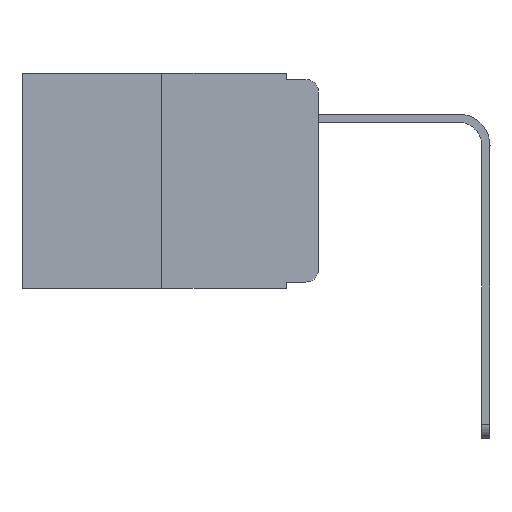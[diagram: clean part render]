
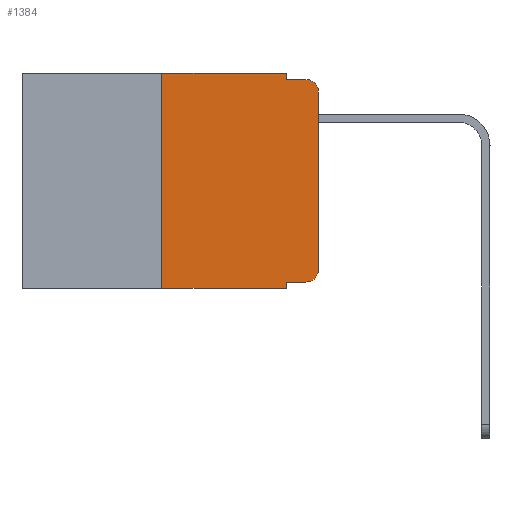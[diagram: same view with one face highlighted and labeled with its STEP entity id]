
A CAD part, left-side view. The second image highlights one B-rep face of the part: STEP entity #1384.
In plain terms, the highlighted planar face has unit normal (-1, 0, 0).
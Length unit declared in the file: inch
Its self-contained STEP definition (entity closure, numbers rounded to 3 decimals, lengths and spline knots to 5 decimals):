
#184 = ORIENTED_EDGE ( 'NONE', *, *, #1946, .T. ) ;
#216 = VERTEX_POINT ( 'NONE', #1196 ) ;
#349 = DIRECTION ( 'NONE',  ( 0., 0., -1. ) ) ;
#419 = CARTESIAN_POINT ( 'NONE',  ( 0., 0.25, 0. ) ) ;
#544 = ORIENTED_EDGE ( 'NONE', *, *, #1931, .F. ) ;
#556 = EDGE_CURVE ( 'NONE', #3804, #8467, #6731, .T. ) ;
#856 = LINE ( 'NONE', #9484, #6596 ) ;
#1089 = CARTESIAN_POINT ( 'NONE',  ( 0., 0., -0.313 ) ) ;
#1102 = DIRECTION ( 'NONE',  ( -1., 0., 0. ) ) ;
#1115 = DIRECTION ( 'NONE',  ( 0., 0., 1. ) ) ;
#1196 = CARTESIAN_POINT ( 'NONE',  ( 0., 0.051, -0.333 ) ) ;
#1223 = CARTESIAN_POINT ( 'NONE',  ( 0., 0.051, -0.01 ) ) ;
#1312 = CARTESIAN_POINT ( 'NONE',  ( 0., 0.25, -0.343 ) ) ;
#1384 = ADVANCED_FACE ( 'NONE', ( #4943 ), #7823, .F. ) ;
#1387 = LINE ( 'NONE', #9319, #8066 ) ;
#1457 = EDGE_CURVE ( 'NONE', #3573, #3804, #7039, .T. ) ;
#1873 = DIRECTION ( 'NONE',  ( 0., 0., -1. ) ) ;
#1931 = EDGE_CURVE ( 'NONE', #4893, #8467, #4245, .T. ) ;
#1946 = EDGE_CURVE ( 'NONE', #6320, #6126, #856, .T. ) ;
#2114 = VECTOR ( 'NONE', #9587, 39.37008 ) ;
#2255 = LINE ( 'NONE', #8440, #7183 ) ;
#2430 = VECTOR ( 'NONE', #4287, 39.37008 ) ;
#3028 = VECTOR ( 'NONE', #3867, 39.37008 ) ;
#3076 = EDGE_CURVE ( 'NONE', #216, #4515, #8195, .T. ) ;
#3193 = VERTEX_POINT ( 'NONE', #8867 ) ;
#3284 = CARTESIAN_POINT ( 'NONE',  ( 0., 0.02, -0.313 ) ) ;
#3522 = EDGE_CURVE ( 'NONE', #3193, #4893, #1387, .T. ) ;
#3533 = ORIENTED_EDGE ( 'NONE', *, *, #5985, .F. ) ;
#3573 = VERTEX_POINT ( 'NONE', #1089 ) ;
#3605 = CARTESIAN_POINT ( 'NONE',  ( 0., 0., -0.03 ) ) ;
#3804 = VERTEX_POINT ( 'NONE', #3605 ) ;
#3867 = DIRECTION ( 'NONE',  ( 0., -1., 0. ) ) ;
#3978 = ORIENTED_EDGE ( 'NONE', *, *, #4857, .F. ) ;
#4219 = DIRECTION ( 'NONE',  ( 0., 0., 1. ) ) ;
#4245 = LINE ( 'NONE', #9513, #2114 ) ;
#4287 = DIRECTION ( 'NONE',  ( 0., -1., 0. ) ) ;
#4418 = CARTESIAN_POINT ( 'NONE',  ( 0., 0.02, -0.333 ) ) ;
#4446 = ORIENTED_EDGE ( 'NONE', *, *, #7745, .T. ) ;
#4467 = ORIENTED_EDGE ( 'NONE', *, *, #3522, .F. ) ;
#4511 = CARTESIAN_POINT ( 'NONE',  ( 0., 0.02, -0.03 ) ) ;
#4515 = VERTEX_POINT ( 'NONE', #4418 ) ;
#4616 = ORIENTED_EDGE ( 'NONE', *, *, #9634, .F. ) ;
#4785 = LINE ( 'NONE', #6127, #3028 ) ;
#4789 = CARTESIAN_POINT ( 'NONE',  ( 0., 0.25, 0. ) ) ;
#4812 = DIRECTION ( 'NONE',  ( 1., 0., 0. ) ) ;
#4857 = EDGE_CURVE ( 'NONE', #6320, #6624, #4986, .T. ) ;
#4861 = CARTESIAN_POINT ( 'NONE',  ( 0., 0.051, -0.343 ) ) ;
#4893 = VERTEX_POINT ( 'NONE', #1223 ) ;
#4932 = CARTESIAN_POINT ( 'NONE',  ( 0., 0., 0. ) ) ;
#4943 = FACE_OUTER_BOUND ( 'NONE', #7488, .T. ) ;
#4986 = LINE ( 'NONE', #419, #6398 ) ;
#5155 = CIRCLE ( 'NONE', #8229, 0.02 ) ;
#5441 = ORIENTED_EDGE ( 'NONE', *, *, #556, .T. ) ;
#5495 = DIRECTION ( 'NONE',  ( 0., 0., -1. ) ) ;
#5796 = DIRECTION ( 'NONE',  ( 0., -1., 0. ) ) ;
#5985 = EDGE_CURVE ( 'NONE', #216, #6126, #2255, .T. ) ;
#6013 = DIRECTION ( 'NONE',  ( -1., 0., 0. ) ) ;
#6126 = VERTEX_POINT ( 'NONE', #4861 ) ;
#6127 = CARTESIAN_POINT ( 'NONE',  ( 0., 0.473, 0. ) ) ;
#6320 = VERTEX_POINT ( 'NONE', #1312 ) ;
#6398 = VECTOR ( 'NONE', #4219, 39.37008 ) ;
#6596 = VECTOR ( 'NONE', #5796, 39.37008 ) ;
#6624 = VERTEX_POINT ( 'NONE', #4789 ) ;
#6731 = CIRCLE ( 'NONE', #8581, 0.02 ) ;
#7039 = LINE ( 'NONE', #4932, #7750 ) ;
#7141 = ORIENTED_EDGE ( 'NONE', *, *, #1457, .T. ) ;
#7183 = VECTOR ( 'NONE', #5495, 39.37008 ) ;
#7189 = CARTESIAN_POINT ( 'NONE',  ( 0., 0.473, 0. ) ) ;
#7211 = CARTESIAN_POINT ( 'NONE',  ( 0., 0.051, -0.333 ) ) ;
#7329 = AXIS2_PLACEMENT_3D ( 'NONE', #7189, #4812, #1873 ) ;
#7488 = EDGE_LOOP ( 'NONE', ( #7141, #5441, #544, #4467, #4616, #3978, #184, #3533, #8170, #4446 ) ) ;
#7506 = DIRECTION ( 'NONE',  ( 0., 0., -1. ) ) ;
#7608 = CARTESIAN_POINT ( 'NONE',  ( 0., 0.02, -0.01 ) ) ;
#7745 = EDGE_CURVE ( 'NONE', #4515, #3573, #5155, .T. ) ;
#7750 = VECTOR ( 'NONE', #1115, 39.37008 ) ;
#7823 = PLANE ( 'NONE',  #7329 ) ;
#8066 = VECTOR ( 'NONE', #349, 39.37008 ) ;
#8170 = ORIENTED_EDGE ( 'NONE', *, *, #3076, .T. ) ;
#8195 = LINE ( 'NONE', #7211, #2430 ) ;
#8229 = AXIS2_PLACEMENT_3D ( 'NONE', #3284, #1102, #9421 ) ;
#8440 = CARTESIAN_POINT ( 'NONE',  ( 0., 0.051, 0. ) ) ;
#8467 = VERTEX_POINT ( 'NONE', #7608 ) ;
#8581 = AXIS2_PLACEMENT_3D ( 'NONE', #4511, #6013, #7506 ) ;
#8867 = CARTESIAN_POINT ( 'NONE',  ( 0., 0.051, 0. ) ) ;
#9319 = CARTESIAN_POINT ( 'NONE',  ( 0., 0.051, 0. ) ) ;
#9421 = DIRECTION ( 'NONE',  ( 0., 0., -1. ) ) ;
#9484 = CARTESIAN_POINT ( 'NONE',  ( 0., 0.473, -0.343 ) ) ;
#9513 = CARTESIAN_POINT ( 'NONE',  ( 0., 0.051, -0.01 ) ) ;
#9587 = DIRECTION ( 'NONE',  ( 0., -1., 0. ) ) ;
#9634 = EDGE_CURVE ( 'NONE', #6624, #3193, #4785, .T. ) ;
